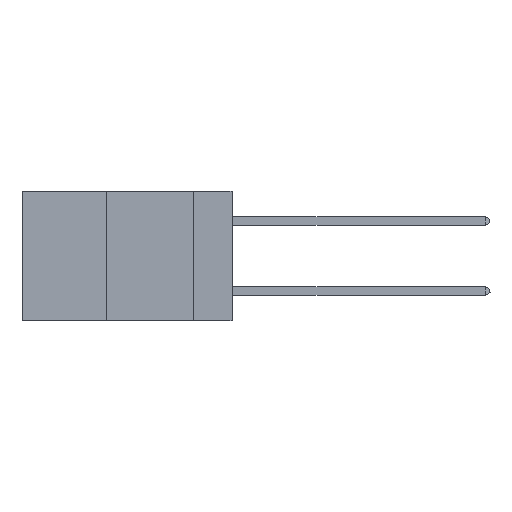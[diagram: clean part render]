
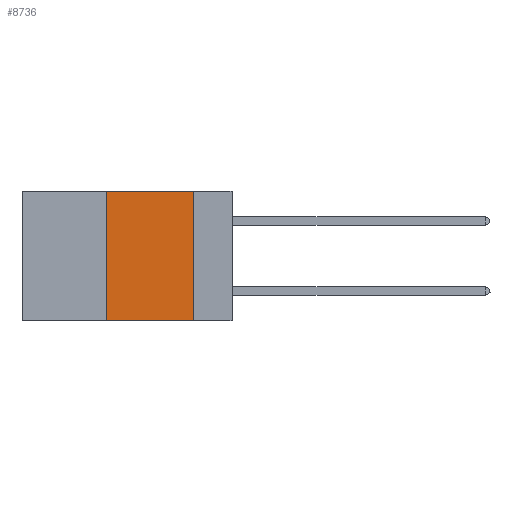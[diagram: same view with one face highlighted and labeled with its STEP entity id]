
A CAD part, left-side view. The second image highlights one B-rep face of the part: STEP entity #8736.
In plain terms, the highlighted planar face has unit normal (-1, 0, 0).
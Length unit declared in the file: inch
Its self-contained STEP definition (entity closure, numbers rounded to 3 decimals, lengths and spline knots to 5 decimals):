
#591 = DIRECTION ( 'NONE',  ( 0., 0., -1. ) ) ;
#976 = CARTESIAN_POINT ( 'NONE',  ( 0., 0.36, 0. ) ) ;
#1606 = DIRECTION ( 'NONE',  ( 0., 0., -1. ) ) ;
#1658 = DIRECTION ( 'NONE',  ( 0., -1., 0. ) ) ;
#1664 = CARTESIAN_POINT ( 'NONE',  ( 0., 0.6, 0. ) ) ;
#2092 = DIRECTION ( 'NONE',  ( 0., 0., 1. ) ) ;
#2818 = CARTESIAN_POINT ( 'NONE',  ( 0., 0.36, 0. ) ) ;
#2859 = CARTESIAN_POINT ( 'NONE',  ( 0., 0.36, -0.37 ) ) ;
#3553 = ORIENTED_EDGE ( 'NONE', *, *, #13025, .F. ) ;
#4125 = VERTEX_POINT ( 'NONE', #13457 ) ;
#5203 = EDGE_CURVE ( 'NONE', #13373, #4125, #13241, .T. ) ;
#6454 = VECTOR ( 'NONE', #1658, 39.37008 ) ;
#6932 = CARTESIAN_POINT ( 'NONE',  ( 0., 0.6, -0.37 ) ) ;
#7108 = CARTESIAN_POINT ( 'NONE',  ( 0., 0.6, 0. ) ) ;
#7217 = FACE_OUTER_BOUND ( 'NONE', #13059, .T. ) ;
#7293 = ORIENTED_EDGE ( 'NONE', *, *, #5203, .T. ) ;
#7548 = EDGE_CURVE ( 'NONE', #14854, #10544, #13624, .T. ) ;
#7621 = EDGE_CURVE ( 'NONE', #10544, #4125, #13830, .T. ) ;
#8736 = ADVANCED_FACE ( 'NONE', ( #7217 ), #9763, .F. ) ;
#9162 = AXIS2_PLACEMENT_3D ( 'NONE', #1664, #16526, #1606 ) ;
#9763 = PLANE ( 'NONE',  #9162 ) ;
#10417 = ORIENTED_EDGE ( 'NONE', *, *, #7621, .F. ) ;
#10544 = VERTEX_POINT ( 'NONE', #16540 ) ;
#10826 = VECTOR ( 'NONE', #591, 39.37008 ) ;
#11284 = LINE ( 'NONE', #2818, #16119 ) ;
#13025 = EDGE_CURVE ( 'NONE', #13373, #14854, #11284, .T. ) ;
#13059 = EDGE_LOOP ( 'NONE', ( #10417, #14509, #3553, #7293 ) ) ;
#13241 = LINE ( 'NONE', #6932, #13466 ) ;
#13373 = VERTEX_POINT ( 'NONE', #2859 ) ;
#13457 = CARTESIAN_POINT ( 'NONE',  ( 0., 0.11, -0.37 ) ) ;
#13466 = VECTOR ( 'NONE', #16404, 39.37008 ) ;
#13624 = LINE ( 'NONE', #7108, #6454 ) ;
#13830 = LINE ( 'NONE', #16809, #10826 ) ;
#14509 = ORIENTED_EDGE ( 'NONE', *, *, #7548, .F. ) ;
#14854 = VERTEX_POINT ( 'NONE', #976 ) ;
#16119 = VECTOR ( 'NONE', #2092, 39.37008 ) ;
#16404 = DIRECTION ( 'NONE',  ( 0., -1., 0. ) ) ;
#16526 = DIRECTION ( 'NONE',  ( 1., 0., 0. ) ) ;
#16540 = CARTESIAN_POINT ( 'NONE',  ( 0., 0.11, 0. ) ) ;
#16809 = CARTESIAN_POINT ( 'NONE',  ( 0., 0.11, 0. ) ) ;
